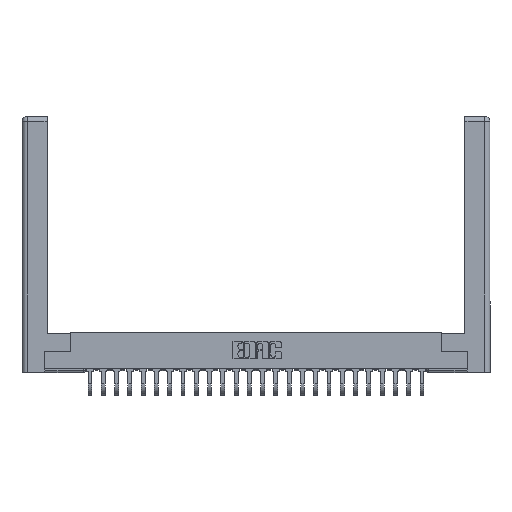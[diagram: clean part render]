
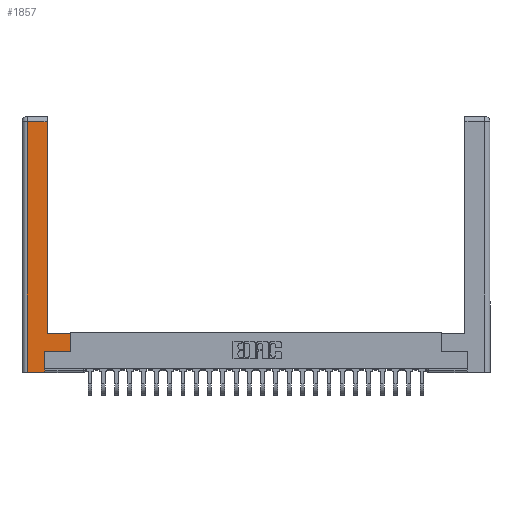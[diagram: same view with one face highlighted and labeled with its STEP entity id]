
A CAD part, top view. The second image highlights one B-rep face of the part: STEP entity #1857.
In plain terms, the highlighted planar face has unit normal (0, 0, 1).
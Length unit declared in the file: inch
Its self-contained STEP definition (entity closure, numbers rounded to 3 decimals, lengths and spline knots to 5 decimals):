
#86 = LINE ( 'NONE', #4460, #7259 ) ;
#915 = CARTESIAN_POINT ( 'NONE',  ( 0.0615, 0., 0. ) ) ;
#998 = VERTEX_POINT ( 'NONE', #5411 ) ;
#1604 = EDGE_CURVE ( 'NONE', #24730, #998, #21199, .T. ) ;
#1623 = PLANE ( 'NONE',  #11675 ) ;
#1857 = ADVANCED_FACE ( 'NONE', ( #8310 ), #1623, .F. ) ;
#2054 = VECTOR ( 'NONE', #16811, 39.37008 ) ;
#2093 = LINE ( 'NONE', #21385, #12542 ) ;
#3716 = DIRECTION ( 'NONE',  ( 1., 0., 0. ) ) ;
#4026 = EDGE_CURVE ( 'NONE', #26027, #24730, #2093, .T. ) ;
#4254 = VERTEX_POINT ( 'NONE', #19932 ) ;
#4460 = CARTESIAN_POINT ( 'NONE',  ( 0.265, 0., 0. ) ) ;
#4485 = ORIENTED_EDGE ( 'NONE', *, *, #24713, .T. ) ;
#4809 = EDGE_CURVE ( 'NONE', #16208, #13575, #6847, .T. ) ;
#4935 = DIRECTION ( 'NONE',  ( 0., -1., 0. ) ) ;
#5411 = CARTESIAN_POINT ( 'NONE',  ( 0.295, 2.94, 0. ) ) ;
#6847 = LINE ( 'NONE', #25432, #9383 ) ;
#7259 = VECTOR ( 'NONE', #26877, 39.37008 ) ;
#7556 = EDGE_LOOP ( 'NONE', ( #11888, #4485, #21632, #12203, #15050, #7774, #13918, #16521 ) ) ;
#7672 = CARTESIAN_POINT ( 'NONE',  ( 0.565, 0.45, 0. ) ) ;
#7694 = EDGE_CURVE ( 'NONE', #4254, #7887, #22333, .T. ) ;
#7774 = ORIENTED_EDGE ( 'NONE', *, *, #15931, .T. ) ;
#7887 = VERTEX_POINT ( 'NONE', #12841 ) ;
#8310 = FACE_OUTER_BOUND ( 'NONE', #7556, .T. ) ;
#8465 = CARTESIAN_POINT ( 'NONE',  ( 0.295, 3., 0. ) ) ;
#9383 = VECTOR ( 'NONE', #4935, 39.37008 ) ;
#9866 = CARTESIAN_POINT ( 'NONE',  ( 0.565, 0.245, 0. ) ) ;
#9879 = DIRECTION ( 'NONE',  ( 0., 1., 0. ) ) ;
#9946 = CARTESIAN_POINT ( 'NONE',  ( 0.0615, 2.94, 0. ) ) ;
#9955 = LINE ( 'NONE', #16513, #13130 ) ;
#10285 = DIRECTION ( 'NONE',  ( -1., 0., 0. ) ) ;
#11481 = LINE ( 'NONE', #23677, #25178 ) ;
#11502 = EDGE_CURVE ( 'NONE', #13575, #4254, #86, .T. ) ;
#11675 = AXIS2_PLACEMENT_3D ( 'NONE', #22544, #22238, #20512 ) ;
#11888 = ORIENTED_EDGE ( 'NONE', *, *, #1604, .T. ) ;
#12203 = ORIENTED_EDGE ( 'NONE', *, *, #11502, .T. ) ;
#12536 = VERTEX_POINT ( 'NONE', #15199 ) ;
#12542 = VECTOR ( 'NONE', #10285, 39.37008 ) ;
#12841 = CARTESIAN_POINT ( 'NONE',  ( 0.265, 0.245, 0. ) ) ;
#13130 = VECTOR ( 'NONE', #22265, 39.37008 ) ;
#13575 = VERTEX_POINT ( 'NONE', #915 ) ;
#13918 = ORIENTED_EDGE ( 'NONE', *, *, #20945, .T. ) ;
#15016 = VECTOR ( 'NONE', #9879, 39.37008 ) ;
#15050 = ORIENTED_EDGE ( 'NONE', *, *, #7694, .T. ) ;
#15199 = CARTESIAN_POINT ( 'NONE',  ( 0.565, 0.245, 0. ) ) ;
#15931 = EDGE_CURVE ( 'NONE', #7887, #12536, #17675, .T. ) ;
#16208 = VERTEX_POINT ( 'NONE', #9946 ) ;
#16389 = VECTOR ( 'NONE', #3716, 39.37008 ) ;
#16513 = CARTESIAN_POINT ( 'NONE',  ( 0.565, 0.45, 0. ) ) ;
#16521 = ORIENTED_EDGE ( 'NONE', *, *, #4026, .T. ) ;
#16811 = DIRECTION ( 'NONE',  ( 0., 1., 0. ) ) ;
#17675 = LINE ( 'NONE', #9866, #16389 ) ;
#17811 = DIRECTION ( 'NONE',  ( -1., 0., 0. ) ) ;
#19932 = CARTESIAN_POINT ( 'NONE',  ( 0.265, 0., 0. ) ) ;
#20512 = DIRECTION ( 'NONE',  ( -1., 0., 0. ) ) ;
#20945 = EDGE_CURVE ( 'NONE', #12536, #26027, #9955, .T. ) ;
#21199 = LINE ( 'NONE', #8465, #2054 ) ;
#21385 = CARTESIAN_POINT ( 'NONE',  ( 0.295, 0.45, 0. ) ) ;
#21632 = ORIENTED_EDGE ( 'NONE', *, *, #4809, .T. ) ;
#22238 = DIRECTION ( 'NONE',  ( 0., 0., -1. ) ) ;
#22265 = DIRECTION ( 'NONE',  ( 0., 1., 0. ) ) ;
#22333 = LINE ( 'NONE', #24645, #15016 ) ;
#22544 = CARTESIAN_POINT ( 'NONE',  ( 0., 0., 0. ) ) ;
#23677 = CARTESIAN_POINT ( 'NONE',  ( 0.0615, 2.94, 0. ) ) ;
#24645 = CARTESIAN_POINT ( 'NONE',  ( 0.265, 0.245, 0. ) ) ;
#24713 = EDGE_CURVE ( 'NONE', #998, #16208, #11481, .T. ) ;
#24730 = VERTEX_POINT ( 'NONE', #25736 ) ;
#25178 = VECTOR ( 'NONE', #17811, 39.37008 ) ;
#25432 = CARTESIAN_POINT ( 'NONE',  ( 0.0615, 0., 0. ) ) ;
#25736 = CARTESIAN_POINT ( 'NONE',  ( 0.295, 0.45, 0. ) ) ;
#26027 = VERTEX_POINT ( 'NONE', #7672 ) ;
#26877 = DIRECTION ( 'NONE',  ( 1., 0., 0. ) ) ;
